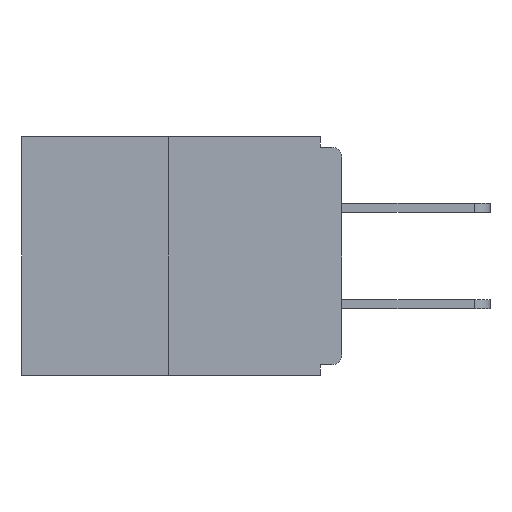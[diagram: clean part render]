
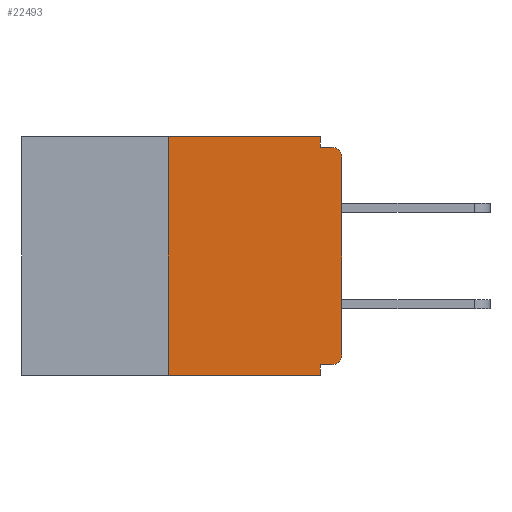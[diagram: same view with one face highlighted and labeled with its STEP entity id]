
A CAD part, left-side view. The second image highlights one B-rep face of the part: STEP entity #22493.
In plain terms, the highlighted planar face has unit normal (-1, 0, 0).
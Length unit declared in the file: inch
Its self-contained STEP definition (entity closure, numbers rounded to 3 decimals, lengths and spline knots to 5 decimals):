
#107 = ORIENTED_EDGE ( 'NONE', *, *, #5355, .F. ) ;
#200 = VERTEX_POINT ( 'NONE', #1038 ) ;
#475 = ORIENTED_EDGE ( 'NONE', *, *, #19131, .T. ) ;
#703 = CARTESIAN_POINT ( 'NONE',  ( 0., 0.031, 0. ) ) ;
#719 = AXIS2_PLACEMENT_3D ( 'NONE', #2630, #4786, #14746 ) ;
#850 = EDGE_CURVE ( 'NONE', #25582, #12038, #19940, .T. ) ;
#1038 = CARTESIAN_POINT ( 'NONE',  ( 0., 0.031, -0.328 ) ) ;
#2124 = ORIENTED_EDGE ( 'NONE', *, *, #850, .T. ) ;
#2239 = VECTOR ( 'NONE', #3349, 39.37008 ) ;
#2252 = CARTESIAN_POINT ( 'NONE',  ( 0., 0.015, -0.328 ) ) ;
#2563 = EDGE_CURVE ( 'NONE', #20167, #21389, #12436, .T. ) ;
#2630 = CARTESIAN_POINT ( 'NONE',  ( 0., 0.46, 0. ) ) ;
#3024 = AXIS2_PLACEMENT_3D ( 'NONE', #17959, #5666, #9710 ) ;
#3349 = DIRECTION ( 'NONE',  ( 0., 1., 0. ) ) ;
#3565 = CARTESIAN_POINT ( 'NONE',  ( 0., 0.25, -0.343 ) ) ;
#3617 = DIRECTION ( 'NONE',  ( 0., 0., -1. ) ) ;
#3840 = EDGE_LOOP ( 'NONE', ( #8360, #107, #21514, #16720, #5094, #2124, #475, #10591, #12513, #13281 ) ) ;
#3964 = CARTESIAN_POINT ( 'NONE',  ( 0., 0., -0.313 ) ) ;
#4248 = DIRECTION ( 'NONE',  ( 0., 0., 1. ) ) ;
#4604 = EDGE_CURVE ( 'NONE', #21389, #9904, #26440, .T. ) ;
#4786 = DIRECTION ( 'NONE',  ( 1., 0., 0. ) ) ;
#4925 = VECTOR ( 'NONE', #21955, 39.37008 ) ;
#5094 = ORIENTED_EDGE ( 'NONE', *, *, #11938, .F. ) ;
#5355 = EDGE_CURVE ( 'NONE', #25420, #8536, #15535, .T. ) ;
#5666 = DIRECTION ( 'NONE',  ( -1., 0., 0. ) ) ;
#5688 = DIRECTION ( 'NONE',  ( 0., -1., 0. ) ) ;
#6706 = VECTOR ( 'NONE', #4248, 39.37008 ) ;
#6779 = CARTESIAN_POINT ( 'NONE',  ( 0., 0.031, -0.343 ) ) ;
#6791 = VECTOR ( 'NONE', #10163, 39.37008 ) ;
#8360 = ORIENTED_EDGE ( 'NONE', *, *, #24506, .F. ) ;
#8536 = VERTEX_POINT ( 'NONE', #24053 ) ;
#8862 = CARTESIAN_POINT ( 'NONE',  ( 0., 0.031, -0.343 ) ) ;
#8870 = EDGE_CURVE ( 'NONE', #25420, #20694, #12656, .T. ) ;
#9097 = CARTESIAN_POINT ( 'NONE',  ( 0., 0., -0.015 ) ) ;
#9710 = DIRECTION ( 'NONE',  ( 0., 0., -1. ) ) ;
#9750 = AXIS2_PLACEMENT_3D ( 'NONE', #23731, #13465, #3617 ) ;
#9755 = CARTESIAN_POINT ( 'NONE',  ( 0., 0.015, -0.015 ) ) ;
#9904 = VERTEX_POINT ( 'NONE', #9755 ) ;
#10146 = VERTEX_POINT ( 'NONE', #19437 ) ;
#10163 = DIRECTION ( 'NONE',  ( 0., 0., 1. ) ) ;
#10427 = CARTESIAN_POINT ( 'NONE',  ( 0., 0.46, 0. ) ) ;
#10591 = ORIENTED_EDGE ( 'NONE', *, *, #17723, .T. ) ;
#11938 = EDGE_CURVE ( 'NONE', #25582, #200, #13152, .T. ) ;
#12038 = VERTEX_POINT ( 'NONE', #3964 ) ;
#12436 = LINE ( 'NONE', #22901, #22084 ) ;
#12513 = ORIENTED_EDGE ( 'NONE', *, *, #4604, .F. ) ;
#12554 = LINE ( 'NONE', #10427, #25429 ) ;
#12558 = DIRECTION ( 'NONE',  ( 0., 0., -1. ) ) ;
#12571 = CARTESIAN_POINT ( 'NONE',  ( 0., 0.25, 0. ) ) ;
#12656 = LINE ( 'NONE', #15218, #4925 ) ;
#12897 = CIRCLE ( 'NONE', #9750, 0.015 ) ;
#13152 = LINE ( 'NONE', #21759, #2239 ) ;
#13281 = ORIENTED_EDGE ( 'NONE', *, *, #2563, .F. ) ;
#13465 = DIRECTION ( 'NONE',  ( -1., 0., 0. ) ) ;
#14746 = DIRECTION ( 'NONE',  ( 0., 0., -1. ) ) ;
#15218 = CARTESIAN_POINT ( 'NONE',  ( 0., 0.46, -0.343 ) ) ;
#15535 = LINE ( 'NONE', #12571, #6791 ) ;
#16424 = DIRECTION ( 'NONE',  ( 0., -1., 0. ) ) ;
#16720 = ORIENTED_EDGE ( 'NONE', *, *, #24150, .F. ) ;
#17723 = EDGE_CURVE ( 'NONE', #10146, #9904, #12897, .T. ) ;
#17959 = CARTESIAN_POINT ( 'NONE',  ( 0., 0.015, -0.313 ) ) ;
#18047 = VECTOR ( 'NONE', #23231, 39.37008 ) ;
#19131 = EDGE_CURVE ( 'NONE', #12038, #10146, #19912, .T. ) ;
#19244 = PLANE ( 'NONE',  #719 ) ;
#19437 = CARTESIAN_POINT ( 'NONE',  ( 0., 0., -0.03 ) ) ;
#19651 = LINE ( 'NONE', #8862, #18047 ) ;
#19912 = LINE ( 'NONE', #24901, #6706 ) ;
#19940 = CIRCLE ( 'NONE', #3024, 0.015 ) ;
#20167 = VERTEX_POINT ( 'NONE', #703 ) ;
#20245 = CARTESIAN_POINT ( 'NONE',  ( 0., 0.031, -0.015 ) ) ;
#20694 = VERTEX_POINT ( 'NONE', #6779 ) ;
#21389 = VERTEX_POINT ( 'NONE', #20245 ) ;
#21514 = ORIENTED_EDGE ( 'NONE', *, *, #8870, .T. ) ;
#21759 = CARTESIAN_POINT ( 'NONE',  ( 0., 0., -0.328 ) ) ;
#21955 = DIRECTION ( 'NONE',  ( 0., -1., 0. ) ) ;
#22084 = VECTOR ( 'NONE', #12558, 39.37008 ) ;
#22334 = FACE_OUTER_BOUND ( 'NONE', #3840, .T. ) ;
#22493 = ADVANCED_FACE ( 'NONE', ( #22334 ), #19244, .F. ) ;
#22901 = CARTESIAN_POINT ( 'NONE',  ( 0., 0.031, 0. ) ) ;
#23231 = DIRECTION ( 'NONE',  ( 0., 0., -1. ) ) ;
#23731 = CARTESIAN_POINT ( 'NONE',  ( 0., 0.015, -0.03 ) ) ;
#24053 = CARTESIAN_POINT ( 'NONE',  ( 0., 0.25, 0. ) ) ;
#24150 = EDGE_CURVE ( 'NONE', #200, #20694, #19651, .T. ) ;
#24506 = EDGE_CURVE ( 'NONE', #8536, #20167, #12554, .T. ) ;
#24901 = CARTESIAN_POINT ( 'NONE',  ( 0., 0., 0. ) ) ;
#25420 = VERTEX_POINT ( 'NONE', #3565 ) ;
#25429 = VECTOR ( 'NONE', #16424, 39.37008 ) ;
#25582 = VERTEX_POINT ( 'NONE', #2252 ) ;
#26145 = VECTOR ( 'NONE', #5688, 39.37008 ) ;
#26440 = LINE ( 'NONE', #9097, #26145 ) ;
